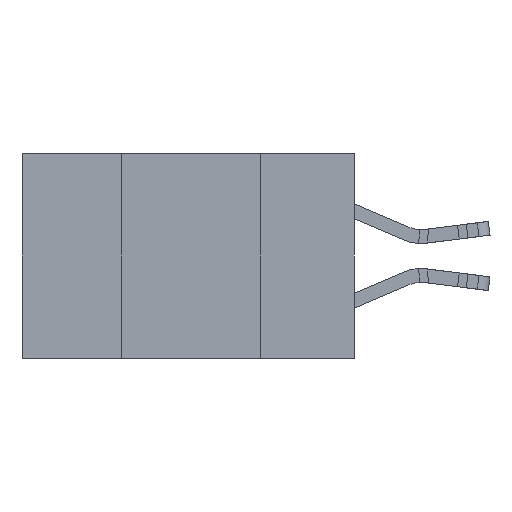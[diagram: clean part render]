
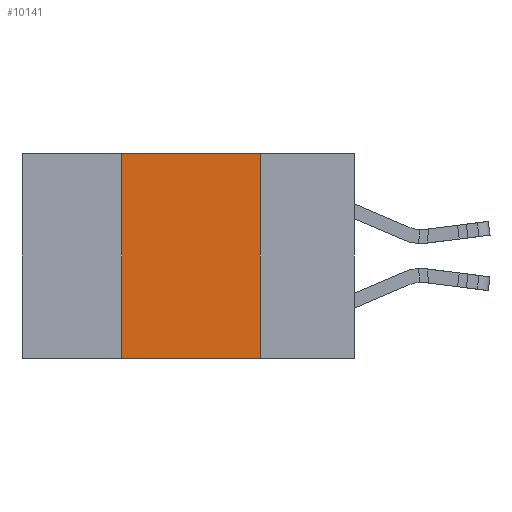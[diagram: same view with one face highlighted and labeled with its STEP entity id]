
A CAD part, left-side view. The second image highlights one B-rep face of the part: STEP entity #10141.
In plain terms, the highlighted planar face has unit normal (-1, 0, 0).
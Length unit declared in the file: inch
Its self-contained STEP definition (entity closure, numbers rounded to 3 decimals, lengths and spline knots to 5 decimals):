
#104 = DIRECTION ( 'NONE',  ( 0., 0., -1. ) ) ;
#899 = EDGE_LOOP ( 'NONE', ( #8080, #8257, #2307, #18640 ) ) ;
#1215 = FACE_OUTER_BOUND ( 'NONE', #899, .T. ) ;
#1663 = VERTEX_POINT ( 'NONE', #24529 ) ;
#1885 = CARTESIAN_POINT ( 'NONE',  ( 0., 0.6, 0. ) ) ;
#2307 = ORIENTED_EDGE ( 'NONE', *, *, #14423, .F. ) ;
#2624 = VERTEX_POINT ( 'NONE', #19495 ) ;
#2779 = DIRECTION ( 'NONE',  ( 0., 0., -1. ) ) ;
#3678 = EDGE_CURVE ( 'NONE', #29501, #1663, #18159, .T. ) ;
#4876 = DIRECTION ( 'NONE',  ( 0., -1., 0. ) ) ;
#7891 = VERTEX_POINT ( 'NONE', #14469 ) ;
#8080 = ORIENTED_EDGE ( 'NONE', *, *, #3678, .F. ) ;
#8257 = ORIENTED_EDGE ( 'NONE', *, *, #8615, .F. ) ;
#8615 = EDGE_CURVE ( 'NONE', #2624, #29501, #12003, .T. ) ;
#10096 = VECTOR ( 'NONE', #2779, 39.37008 ) ;
#10141 = ADVANCED_FACE ( 'NONE', ( #1215 ), #27200, .F. ) ;
#10267 = VECTOR ( 'NONE', #26177, 39.37008 ) ;
#10757 = AXIS2_PLACEMENT_3D ( 'NONE', #12652, #15125, #104 ) ;
#11942 = DIRECTION ( 'NONE',  ( 0., -1., 0. ) ) ;
#12003 = LINE ( 'NONE', #1885, #31274 ) ;
#12480 = CARTESIAN_POINT ( 'NONE',  ( 0., 0.6, -0.37 ) ) ;
#12652 = CARTESIAN_POINT ( 'NONE',  ( 0., 0.6, 0. ) ) ;
#14423 = EDGE_CURVE ( 'NONE', #7891, #2624, #30382, .T. ) ;
#14469 = CARTESIAN_POINT ( 'NONE',  ( 0., 0.42, -0.37 ) ) ;
#15125 = DIRECTION ( 'NONE',  ( 1., 0., 0. ) ) ;
#18159 = LINE ( 'NONE', #30469, #10096 ) ;
#18640 = ORIENTED_EDGE ( 'NONE', *, *, #31738, .T. ) ;
#19495 = CARTESIAN_POINT ( 'NONE',  ( 0., 0.42, 0. ) ) ;
#19971 = CARTESIAN_POINT ( 'NONE',  ( 0., 0.17, 0. ) ) ;
#20816 = VECTOR ( 'NONE', #4876, 39.37008 ) ;
#24529 = CARTESIAN_POINT ( 'NONE',  ( 0., 0.17, -0.37 ) ) ;
#26078 = CARTESIAN_POINT ( 'NONE',  ( 0., 0.42, 0. ) ) ;
#26177 = DIRECTION ( 'NONE',  ( 0., 0., 1. ) ) ;
#27200 = PLANE ( 'NONE',  #10757 ) ;
#28011 = LINE ( 'NONE', #12480, #20816 ) ;
#29501 = VERTEX_POINT ( 'NONE', #19971 ) ;
#30382 = LINE ( 'NONE', #26078, #10267 ) ;
#30469 = CARTESIAN_POINT ( 'NONE',  ( 0., 0.17, 0. ) ) ;
#31274 = VECTOR ( 'NONE', #11942, 39.37008 ) ;
#31738 = EDGE_CURVE ( 'NONE', #7891, #1663, #28011, .T. ) ;
